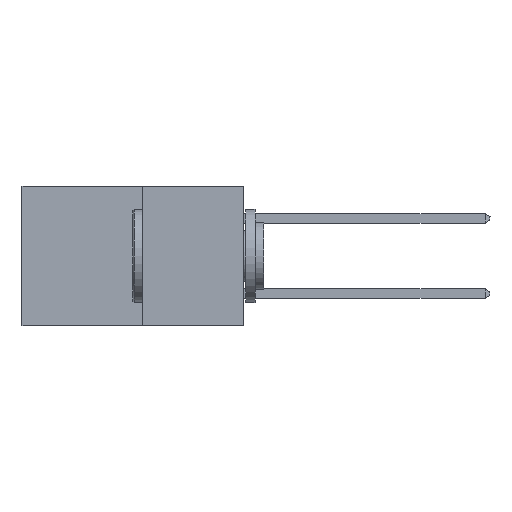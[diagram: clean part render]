
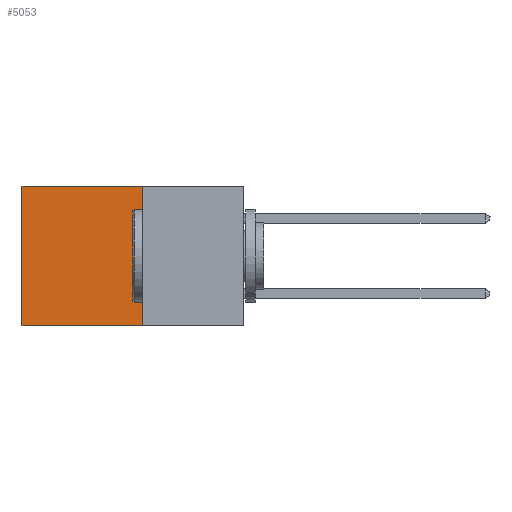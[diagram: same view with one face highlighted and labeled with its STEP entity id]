
A CAD part, left-side view. The second image highlights one B-rep face of the part: STEP entity #5053.
In plain terms, the highlighted planar face has unit normal (-1, 0, 0).
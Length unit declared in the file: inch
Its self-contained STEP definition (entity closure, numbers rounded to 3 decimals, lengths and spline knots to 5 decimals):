
#622 = AXIS2_PLACEMENT_3D ( 'NONE', #20125, #7177, #20052 ) ;
#1129 = VECTOR ( 'NONE', #12914, 39.37008 ) ;
#1396 = DIRECTION ( 'NONE',  ( 0., 1., 0. ) ) ;
#1676 = LINE ( 'NONE', #11368, #1129 ) ;
#2258 = LINE ( 'NONE', #4464, #6126 ) ;
#2560 = DIRECTION ( 'NONE',  ( 0., 1., 0. ) ) ;
#3054 = ORIENTED_EDGE ( 'NONE', *, *, #8559, .F. ) ;
#3845 = ORIENTED_EDGE ( 'NONE', *, *, #17567, .F. ) ;
#4176 = VERTEX_POINT ( 'NONE', #14202 ) ;
#4464 = CARTESIAN_POINT ( 'NONE',  ( 0.277, 0.27, -0.37 ) ) ;
#5053 = ADVANCED_FACE ( 'NONE', ( #9075 ), #13163, .F. ) ;
#5382 = EDGE_LOOP ( 'NONE', ( #5629, #3054, #3845, #12580 ) ) ;
#5629 = ORIENTED_EDGE ( 'NONE', *, *, #11072, .T. ) ;
#6126 = VECTOR ( 'NONE', #1396, 39.37008 ) ;
#6148 = CARTESIAN_POINT ( 'NONE',  ( 0.277, 0.59, 0. ) ) ;
#6584 = VECTOR ( 'NONE', #2560, 39.37008 ) ;
#7177 = DIRECTION ( 'NONE',  ( 1., 0., 0. ) ) ;
#7236 = VERTEX_POINT ( 'NONE', #19089 ) ;
#8046 = LINE ( 'NONE', #16403, #19757 ) ;
#8559 = EDGE_CURVE ( 'NONE', #9118, #4176, #2258, .T. ) ;
#9075 = FACE_OUTER_BOUND ( 'NONE', #5382, .T. ) ;
#9118 = VERTEX_POINT ( 'NONE', #15525 ) ;
#11072 = EDGE_CURVE ( 'NONE', #15910, #4176, #8046, .T. ) ;
#11368 = CARTESIAN_POINT ( 'NONE',  ( 0.277, 0.27, -0.37 ) ) ;
#12580 = ORIENTED_EDGE ( 'NONE', *, *, #17939, .T. ) ;
#12914 = DIRECTION ( 'NONE',  ( 0., 0., -1. ) ) ;
#13163 = PLANE ( 'NONE',  #622 ) ;
#13857 = CARTESIAN_POINT ( 'NONE',  ( 0.277, 0.27, 0. ) ) ;
#14202 = CARTESIAN_POINT ( 'NONE',  ( 0.277, 0.59, -0.37 ) ) ;
#15060 = LINE ( 'NONE', #13857, #6584 ) ;
#15525 = CARTESIAN_POINT ( 'NONE',  ( 0.277, 0.27, -0.37 ) ) ;
#15910 = VERTEX_POINT ( 'NONE', #6148 ) ;
#16160 = DIRECTION ( 'NONE',  ( 0., 0., -1. ) ) ;
#16403 = CARTESIAN_POINT ( 'NONE',  ( 0.277, 0.59, -0.37 ) ) ;
#17567 = EDGE_CURVE ( 'NONE', #7236, #9118, #1676, .T. ) ;
#17939 = EDGE_CURVE ( 'NONE', #7236, #15910, #15060, .T. ) ;
#19089 = CARTESIAN_POINT ( 'NONE',  ( 0.277, 0.27, 0. ) ) ;
#19757 = VECTOR ( 'NONE', #16160, 39.37008 ) ;
#20052 = DIRECTION ( 'NONE',  ( 0., 0., -1. ) ) ;
#20125 = CARTESIAN_POINT ( 'NONE',  ( 0.277, 0.27, -0.37 ) ) ;
